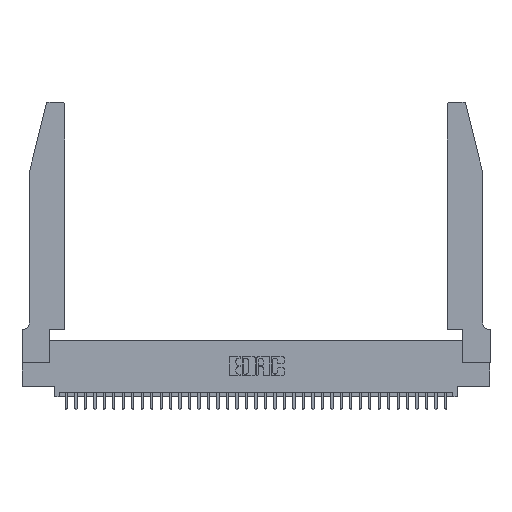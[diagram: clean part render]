
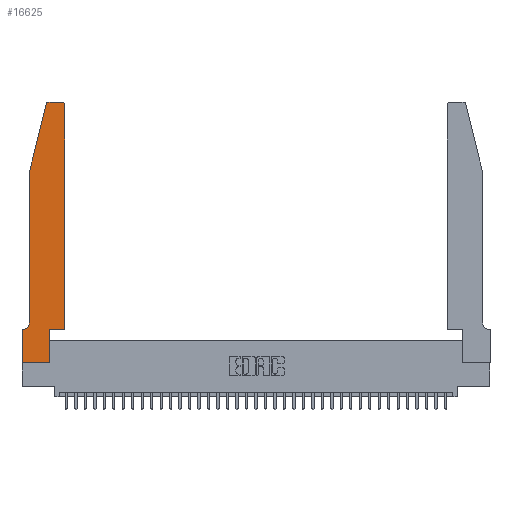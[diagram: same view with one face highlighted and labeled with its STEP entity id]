
A CAD part, top view. The second image highlights one B-rep face of the part: STEP entity #16625.
In plain terms, the highlighted planar face has unit normal (0, 0, 1).
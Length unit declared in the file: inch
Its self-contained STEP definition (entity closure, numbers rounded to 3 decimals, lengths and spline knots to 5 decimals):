
#1549 = DIRECTION ( 'NONE',  ( 0., 1., 0. ) ) ;
#1627 = CARTESIAN_POINT ( 'NONE',  ( 0.4505, 2.72, 0.37 ) ) ;
#1756 = CARTESIAN_POINT ( 'NONE',  ( 0., 0.35, 0.37 ) ) ;
#1783 = ORIENTED_EDGE ( 'NONE', *, *, #22829, .T. ) ;
#1850 = CARTESIAN_POINT ( 'NONE',  ( 0.0755, 2., 0.37 ) ) ;
#2754 = CARTESIAN_POINT ( 'NONE',  ( 0.0055, 0.35, 0.37 ) ) ;
#2759 = EDGE_LOOP ( 'NONE', ( #31390, #36365, #32853, #6215, #12853, #9585, #17518, #17031, #3200, #23318, #19869, #1783 ) ) ;
#2941 = DIRECTION ( 'NONE',  ( 1., 0., 0. ) ) ;
#3120 = EDGE_CURVE ( 'NONE', #28941, #20176, #24351, .T. ) ;
#3200 = ORIENTED_EDGE ( 'NONE', *, *, #11941, .T. ) ;
#3488 = LINE ( 'NONE', #6627, #19683 ) ;
#4110 = FACE_OUTER_BOUND ( 'NONE', #2759, .T. ) ;
#4126 = VECTOR ( 'NONE', #10221, 39.37008 ) ;
#4483 = CIRCLE ( 'NONE', #21593, 0.07 ) ;
#5484 = CARTESIAN_POINT ( 'NONE',  ( 0.0055, 0.42, 0.37 ) ) ;
#5531 = DIRECTION ( 'NONE',  ( 0., 1., 0. ) ) ;
#6192 = LINE ( 'NONE', #31335, #27336 ) ;
#6215 = ORIENTED_EDGE ( 'NONE', *, *, #36835, .T. ) ;
#6269 = EDGE_CURVE ( 'NONE', #7189, #24909, #3488, .T. ) ;
#6627 = CARTESIAN_POINT ( 'NONE',  ( 0.0755, 2., 0.37 ) ) ;
#7189 = VERTEX_POINT ( 'NONE', #31081 ) ;
#7578 = CARTESIAN_POINT ( 'NONE',  ( 0.4505, 0.35, 0.37 ) ) ;
#7640 = VERTEX_POINT ( 'NONE', #1627 ) ;
#9585 = ORIENTED_EDGE ( 'NONE', *, *, #10692, .T. ) ;
#10028 = DIRECTION ( 'NONE',  ( 1., 0., 0. ) ) ;
#10031 = VERTEX_POINT ( 'NONE', #31774 ) ;
#10111 = CIRCLE ( 'NONE', #30469, 0.03 ) ;
#10221 = DIRECTION ( 'NONE',  ( 1., 0., 0. ) ) ;
#10692 = EDGE_CURVE ( 'NONE', #22609, #27748, #23916, .T. ) ;
#10706 = LINE ( 'NONE', #22970, #21942 ) ;
#11941 = EDGE_CURVE ( 'NONE', #18946, #28941, #33696, .T. ) ;
#11957 = AXIS2_PLACEMENT_3D ( 'NONE', #23887, #26569, #35196 ) ;
#12612 = VERTEX_POINT ( 'NONE', #22220 ) ;
#12782 = DIRECTION ( 'NONE',  ( -0.239, -0.971, 0. ) ) ;
#12805 = EDGE_CURVE ( 'NONE', #27748, #10031, #10706, .T. ) ;
#12853 = ORIENTED_EDGE ( 'NONE', *, *, #18271, .T. ) ;
#14041 = DIRECTION ( 'NONE',  ( 0., 0., -1. ) ) ;
#14465 = VERTEX_POINT ( 'NONE', #36652 ) ;
#15025 = VECTOR ( 'NONE', #34011, 39.37008 ) ;
#15174 = VERTEX_POINT ( 'NONE', #23005 ) ;
#15438 = AXIS2_PLACEMENT_3D ( 'NONE', #21230, #15942, #10028 ) ;
#15578 = LINE ( 'NONE', #28862, #16899 ) ;
#15942 = DIRECTION ( 'NONE',  ( 0., 0., 1. ) ) ;
#16289 = VECTOR ( 'NONE', #22956, 39.37008 ) ;
#16625 = ADVANCED_FACE ( 'NONE', ( #4110 ), #21362, .T. ) ;
#16899 = VECTOR ( 'NONE', #2941, 39.37008 ) ;
#16967 = CARTESIAN_POINT ( 'NONE',  ( 0.2865, 0.35, 0.37 ) ) ;
#17031 = ORIENTED_EDGE ( 'NONE', *, *, #25986, .T. ) ;
#17518 = ORIENTED_EDGE ( 'NONE', *, *, #12805, .T. ) ;
#17563 = CIRCLE ( 'NONE', #15438, 0.03 ) ;
#18271 = EDGE_CURVE ( 'NONE', #12612, #22609, #4483, .T. ) ;
#18645 = CARTESIAN_POINT ( 'NONE',  ( 0.2865, 0.35, 0.37 ) ) ;
#18946 = VERTEX_POINT ( 'NONE', #33713 ) ;
#19683 = VECTOR ( 'NONE', #12782, 39.37008 ) ;
#19689 = DIRECTION ( 'NONE',  ( 1., 0., 0. ) ) ;
#19869 = ORIENTED_EDGE ( 'NONE', *, *, #20590, .T. ) ;
#19936 = DIRECTION ( 'NONE',  ( 0., 0., 1. ) ) ;
#20053 = CARTESIAN_POINT ( 'NONE',  ( 0.284, 2.72, 0.37 ) ) ;
#20176 = VERTEX_POINT ( 'NONE', #25866 ) ;
#20590 = EDGE_CURVE ( 'NONE', #20176, #7640, #29477, .T. ) ;
#21230 = CARTESIAN_POINT ( 'NONE',  ( 0.4205, 2.72, 0.37 ) ) ;
#21362 = PLANE ( 'NONE',  #11957 ) ;
#21593 = AXIS2_PLACEMENT_3D ( 'NONE', #5484, #14041, #25471 ) ;
#21750 = LINE ( 'NONE', #1850, #15025 ) ;
#21942 = VECTOR ( 'NONE', #22846, 39.37008 ) ;
#22220 = CARTESIAN_POINT ( 'NONE',  ( 0.0755, 0.42, 0.37 ) ) ;
#22609 = VERTEX_POINT ( 'NONE', #2754 ) ;
#22829 = EDGE_CURVE ( 'NONE', #7640, #15174, #17563, .T. ) ;
#22846 = DIRECTION ( 'NONE',  ( 0., -1., 0. ) ) ;
#22956 = DIRECTION ( 'NONE',  ( -1., 0., 0. ) ) ;
#22970 = CARTESIAN_POINT ( 'NONE',  ( 0., 0., 0.37 ) ) ;
#23005 = CARTESIAN_POINT ( 'NONE',  ( 0.4205, 2.75, 0.37 ) ) ;
#23318 = ORIENTED_EDGE ( 'NONE', *, *, #3120, .T. ) ;
#23887 = CARTESIAN_POINT ( 'NONE',  ( 0., 0.35, 0.37 ) ) ;
#23916 = LINE ( 'NONE', #28614, #16289 ) ;
#24351 = LINE ( 'NONE', #7578, #4126 ) ;
#24909 = VERTEX_POINT ( 'NONE', #33049 ) ;
#25471 = DIRECTION ( 'NONE',  ( -1., 0., 0. ) ) ;
#25866 = CARTESIAN_POINT ( 'NONE',  ( 0.4505, 0.35, 0.37 ) ) ;
#25986 = EDGE_CURVE ( 'NONE', #10031, #18946, #15578, .T. ) ;
#26569 = DIRECTION ( 'NONE',  ( 0., 0., 1. ) ) ;
#27336 = VECTOR ( 'NONE', #36740, 39.37008 ) ;
#27748 = VERTEX_POINT ( 'NONE', #1756 ) ;
#27875 = VECTOR ( 'NONE', #5531, 39.37008 ) ;
#28497 = EDGE_CURVE ( 'NONE', #14465, #7189, #10111, .T. ) ;
#28560 = VECTOR ( 'NONE', #1549, 39.37008 ) ;
#28614 = CARTESIAN_POINT ( 'NONE',  ( 0.0755, 0.35, 0.37 ) ) ;
#28862 = CARTESIAN_POINT ( 'NONE',  ( 0., 0., 0.37 ) ) ;
#28941 = VERTEX_POINT ( 'NONE', #18645 ) ;
#29477 = LINE ( 'NONE', #35985, #28560 ) ;
#30469 = AXIS2_PLACEMENT_3D ( 'NONE', #20053, #19936, #19689 ) ;
#31081 = CARTESIAN_POINT ( 'NONE',  ( 0.25487, 2.72718, 0.37 ) ) ;
#31335 = CARTESIAN_POINT ( 'NONE',  ( 0.2605, 2.75, 0.37 ) ) ;
#31390 = ORIENTED_EDGE ( 'NONE', *, *, #35202, .T. ) ;
#31774 = CARTESIAN_POINT ( 'NONE',  ( 0., 0., 0.37 ) ) ;
#32853 = ORIENTED_EDGE ( 'NONE', *, *, #6269, .T. ) ;
#33049 = CARTESIAN_POINT ( 'NONE',  ( 0.0755, 2., 0.37 ) ) ;
#33696 = LINE ( 'NONE', #16967, #27875 ) ;
#33713 = CARTESIAN_POINT ( 'NONE',  ( 0.2865, 0., 0.37 ) ) ;
#34011 = DIRECTION ( 'NONE',  ( 0., -1., 0. ) ) ;
#35196 = DIRECTION ( 'NONE',  ( 1., 0., 0. ) ) ;
#35202 = EDGE_CURVE ( 'NONE', #15174, #14465, #6192, .T. ) ;
#35985 = CARTESIAN_POINT ( 'NONE',  ( 0.4505, 0.35, 0.37 ) ) ;
#36365 = ORIENTED_EDGE ( 'NONE', *, *, #28497, .T. ) ;
#36652 = CARTESIAN_POINT ( 'NONE',  ( 0.284, 2.75, 0.37 ) ) ;
#36740 = DIRECTION ( 'NONE',  ( -1., 0., 0. ) ) ;
#36835 = EDGE_CURVE ( 'NONE', #24909, #12612, #21750, .T. ) ;
